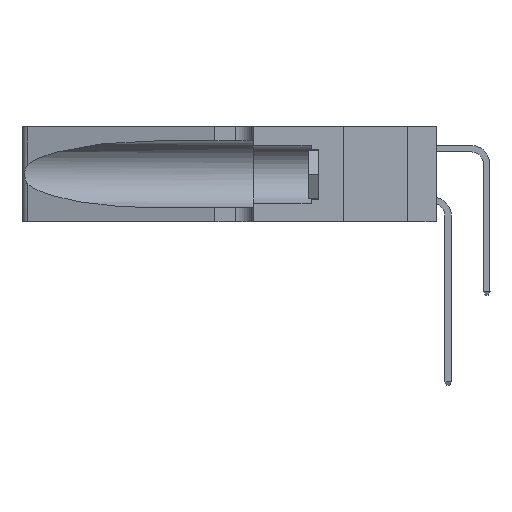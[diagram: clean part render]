
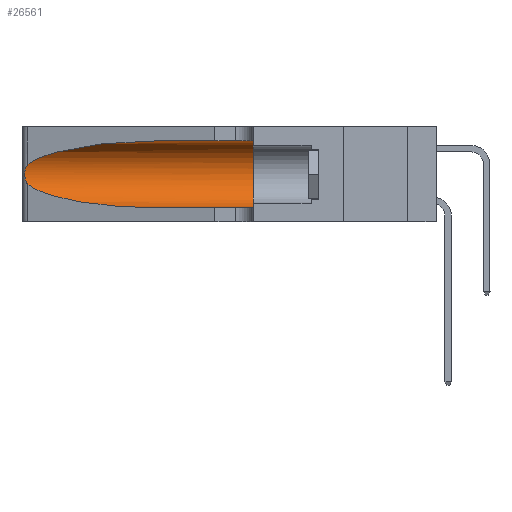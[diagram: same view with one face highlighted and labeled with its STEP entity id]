
A CAD part, left-side view. The second image highlights one B-rep face of the part: STEP entity #26561.
In plain terms, the highlighted cylindrical face has radius 3.308 mm (diameter 6.617 mm), a partial arc.
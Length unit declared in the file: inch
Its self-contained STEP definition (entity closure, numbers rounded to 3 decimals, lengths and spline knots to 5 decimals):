
#1028 = ORIENTED_EDGE ( 'NONE', *, *, #33900, .F. ) ;
#1197 = CARTESIAN_POINT ( 'NONE',  ( 0.1305, 0.72297, 0.31525 ) ) ;
#1889 = VERTEX_POINT ( 'NONE', #24545 ) ;
#2165 = ORIENTED_EDGE ( 'NONE', *, *, #4528, .T. ) ;
#2341 = CARTESIAN_POINT ( 'NONE',  ( 0.26075, 1.23896, 0.19203 ) ) ;
#3677 = VERTEX_POINT ( 'NONE', #26000 ) ;
#3913 = DIRECTION ( 'NONE',  ( 0., -1., 0. ) ) ;
#4122 = EDGE_CURVE ( 'NONE', #1889, #5280, #11228, .T. ) ;
#4291 = VERTEX_POINT ( 'NONE', #34717 ) ;
#4528 = EDGE_CURVE ( 'NONE', #4291, #31488, #31124, .T. ) ;
#4691 = EDGE_LOOP ( 'NONE', ( #2165, #31410, #10781, #35887, #27750, #1028 ) ) ;
#4973 = VECTOR ( 'NONE', #36160, 39.37008 ) ;
#5255 = CARTESIAN_POINT ( 'NONE',  ( 0.1305, 0.72297, 0.05475 ) ) ;
#5280 = VERTEX_POINT ( 'NONE', #27240 ) ;
#6200 =( BOUNDED_CURVE ( )  B_SPLINE_CURVE ( 3, ( #30361, #10584, #11633, #5255 ),
 .UNSPECIFIED., .F., .F. ) 
 B_SPLINE_CURVE_WITH_KNOTS ( ( 4, 4 ),
 ( 3.44316, 4.71239 ),
 .UNSPECIFIED. ) 
 CURVE ( )  GEOMETRIC_REPRESENTATION_ITEM ( )  RATIONAL_B_SPLINE_CURVE ( ( 1., 0.87, 0.87, 1. ) ) 
 REPRESENTATION_ITEM ( '' )  );
#8132 = CARTESIAN_POINT ( 'NONE',  ( 0.25487, 1.22718, 0.14631 ) ) ;
#8327 = CARTESIAN_POINT ( 'NONE',  ( 0.25487, 1.22718, 0.22369 ) ) ;
#8665 = CARTESIAN_POINT ( 'NONE',  ( 0.18966, 0.96281, 0.31525 ) ) ;
#8982 = CARTESIAN_POINT ( 'NONE',  ( 0.26075, 1.23896, 0.178 ) ) ;
#9121 = CARTESIAN_POINT ( 'NONE',  ( 0.25555, 1.22993, 0.14849 ) ) ;
#9283 = DIRECTION ( 'NONE',  ( 0., 0., -1. ) ) ;
#9454 = B_SPLINE_CURVE_WITH_KNOTS ( 'NONE', 3,
 ( #11738, #27580, #40945, #34874, #34301, #21099, #2341, #8982, #28892, #15620, #35568, #41679, #9121, #32098 ),
 .UNSPECIFIED., .F., .F.,
 ( 4, 2, 2, 2, 2, 2, 4 ),
 ( 0., 0.00027, 0.00053, 0.00107, 0.0016, 0.00187, 0.00214 ),
 .UNSPECIFIED. ) ;
#10131 = LINE ( 'NONE', #30504, #29835 ) ;
#10584 = CARTESIAN_POINT ( 'NONE',  ( 0.2373, 1.15595, 0.08982 ) ) ;
#10781 = ORIENTED_EDGE ( 'NONE', *, *, #27852, .T. ) ;
#11228 = LINE ( 'NONE', #25982, #4973 ) ;
#11443 = VERTEX_POINT ( 'NONE', #8132 ) ;
#11633 = CARTESIAN_POINT ( 'NONE',  ( 0.18966, 0.96281, 0.05475 ) ) ;
#11738 = CARTESIAN_POINT ( 'NONE',  ( 0.25487, 1.22718, 0.22369 ) ) ;
#12607 = CARTESIAN_POINT ( 'NONE',  ( 0.1305, 1.61858, 0.185 ) ) ;
#14253 = CARTESIAN_POINT ( 'NONE',  ( 0.2373, 1.15595, 0.28018 ) ) ;
#15620 = CARTESIAN_POINT ( 'NONE',  ( 0.25856, 1.23593, 0.16098 ) ) ;
#16701 = DIRECTION ( 'NONE',  ( 0., 0., 1. ) ) ;
#17206 = AXIS2_PLACEMENT_3D ( 'NONE', #26762, #40392, #16701 ) ;
#19565 = EDGE_CURVE ( 'NONE', #31488, #11443, #9454, .T. ) ;
#21099 = CARTESIAN_POINT ( 'NONE',  ( 0.26018, 1.23835, 0.19895 ) ) ;
#21103 = DIRECTION ( 'NONE',  ( 0., -1., 0. ) ) ;
#21131 = CIRCLE ( 'NONE', #17206, 0.13025 ) ;
#24545 = CARTESIAN_POINT ( 'NONE',  ( 0.1305, 0.72297, 0.05475 ) ) ;
#25982 = CARTESIAN_POINT ( 'NONE',  ( 0.1305, 1.61858, 0.05475 ) ) ;
#26000 = CARTESIAN_POINT ( 'NONE',  ( 0.1305, 0.35, 0.31525 ) ) ;
#26561 = ADVANCED_FACE ( 'NONE', ( #28986 ), #32116, .F. ) ;
#26762 = CARTESIAN_POINT ( 'NONE',  ( 0.1305, 0.35, 0.185 ) ) ;
#27240 = CARTESIAN_POINT ( 'NONE',  ( 0.1305, 0.35, 0.05475 ) ) ;
#27580 = CARTESIAN_POINT ( 'NONE',  ( 0.25555, 1.22994, 0.2215 ) ) ;
#27750 = ORIENTED_EDGE ( 'NONE', *, *, #41150, .F. ) ;
#27852 = EDGE_CURVE ( 'NONE', #11443, #1889, #6200, .T. ) ;
#28892 = CARTESIAN_POINT ( 'NONE',  ( 0.26017, 1.23833, 0.17102 ) ) ;
#28986 = FACE_OUTER_BOUND ( 'NONE', #4691, .T. ) ;
#29835 = VECTOR ( 'NONE', #21103, 39.37008 ) ;
#30361 = CARTESIAN_POINT ( 'NONE',  ( 0.25487, 1.22718, 0.14631 ) ) ;
#30504 = CARTESIAN_POINT ( 'NONE',  ( 0.1305, 1.61858, 0.31525 ) ) ;
#31124 =( BOUNDED_CURVE ( )  B_SPLINE_CURVE ( 3, ( #1197, #8665, #14253, #8327 ),
 .UNSPECIFIED., .F., .T. ) 
 B_SPLINE_CURVE_WITH_KNOTS ( ( 4, 4 ),
 ( 1.5708, 2.84003 ),
 .UNSPECIFIED. ) 
 CURVE ( )  GEOMETRIC_REPRESENTATION_ITEM ( )  RATIONAL_B_SPLINE_CURVE ( ( 1., 0.87, 0.87, 1. ) ) 
 REPRESENTATION_ITEM ( '' )  );
#31346 = CARTESIAN_POINT ( 'NONE',  ( 0.25487, 1.22718, 0.22369 ) ) ;
#31410 = ORIENTED_EDGE ( 'NONE', *, *, #19565, .T. ) ;
#31488 = VERTEX_POINT ( 'NONE', #31346 ) ;
#32098 = CARTESIAN_POINT ( 'NONE',  ( 0.25487, 1.22718, 0.14631 ) ) ;
#32116 = CYLINDRICAL_SURFACE ( 'NONE', #37459, 0.13025 ) ;
#33900 = EDGE_CURVE ( 'NONE', #4291, #3677, #10131, .T. ) ;
#34301 = CARTESIAN_POINT ( 'NONE',  ( 0.25854, 1.2359, 0.20912 ) ) ;
#34717 = CARTESIAN_POINT ( 'NONE',  ( 0.1305, 0.72297, 0.31525 ) ) ;
#34874 = CARTESIAN_POINT ( 'NONE',  ( 0.25787, 1.23484, 0.2124 ) ) ;
#35568 = CARTESIAN_POINT ( 'NONE',  ( 0.25789, 1.23486, 0.15765 ) ) ;
#35887 = ORIENTED_EDGE ( 'NONE', *, *, #4122, .T. ) ;
#36160 = DIRECTION ( 'NONE',  ( 0., -1., 0. ) ) ;
#37459 = AXIS2_PLACEMENT_3D ( 'NONE', #12607, #3913, #9283 ) ;
#40392 = DIRECTION ( 'NONE',  ( 0., 1., 0. ) ) ;
#40945 = CARTESIAN_POINT ( 'NONE',  ( 0.25639, 1.23184, 0.21858 ) ) ;
#41150 = EDGE_CURVE ( 'NONE', #3677, #5280, #21131, .T. ) ;
#41679 = CARTESIAN_POINT ( 'NONE',  ( 0.25639, 1.23186, 0.15144 ) ) ;
